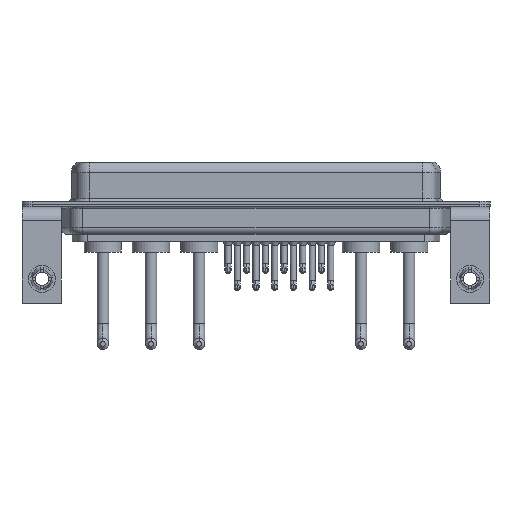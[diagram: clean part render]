
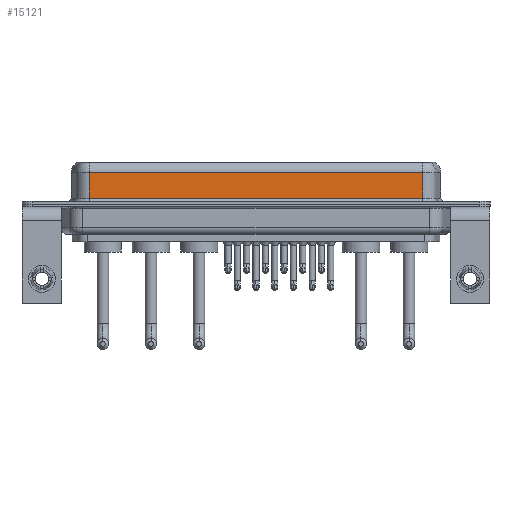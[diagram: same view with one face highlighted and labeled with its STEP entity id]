
A CAD part, front view. The second image highlights one B-rep face of the part: STEP entity #15121.
In plain terms, the highlighted planar face has unit normal (0, -1, 0).
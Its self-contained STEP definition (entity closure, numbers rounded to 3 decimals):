
#917 = FACE_OUTER_BOUND ( 'NONE', #13587, .T. ) ;
#1023 = VERTEX_POINT ( 'NONE', #16857 ) ;
#1134 = DIRECTION ( 'NONE',  ( 0., 1., 0. ) ) ;
#1253 = DIRECTION ( 'NONE',  ( 1., 0., 0. ) ) ;
#2992 = ORIENTED_EDGE ( 'NONE', *, *, #10327, .T. ) ;
#4061 = ORIENTED_EDGE ( 'NONE', *, *, #21674, .T. ) ;
#4792 = EDGE_CURVE ( 'NONE', #5984, #1023, #22410, .T. ) ;
#5480 = LINE ( 'NONE', #7325, #22406 ) ;
#5984 = VERTEX_POINT ( 'NONE', #9066 ) ;
#6277 = ORIENTED_EDGE ( 'NONE', *, *, #4792, .T. ) ;
#6581 = DIRECTION ( 'NONE',  ( -1., 0., 0. ) ) ;
#6910 = VECTOR ( 'NONE', #1253, 1000. ) ;
#7325 = CARTESIAN_POINT ( 'NONE',  ( 7.038, -3.95, 6.4 ) ) ;
#7396 = VERTEX_POINT ( 'NONE', #12749 ) ;
#7765 = PLANE ( 'NONE',  #15214 ) ;
#9066 = CARTESIAN_POINT ( 'NONE',  ( 7.038, -3.95, 0.9 ) ) ;
#10327 = EDGE_CURVE ( 'NONE', #20169, #7396, #18298, .T. ) ;
#10400 = VECTOR ( 'NONE', #19873, 1000. ) ;
#11409 = CARTESIAN_POINT ( 'NONE',  ( 56.462, -3.95, 4.65 ) ) ;
#11547 = CARTESIAN_POINT ( 'NONE',  ( 56.462, -3.95, 0.9 ) ) ;
#11805 = CARTESIAN_POINT ( 'NONE',  ( 56.462, -3.95, 4.65 ) ) ;
#12749 = CARTESIAN_POINT ( 'NONE',  ( 7.038, -3.95, 4.65 ) ) ;
#12929 = CARTESIAN_POINT ( 'NONE',  ( 56.462, -3.95, 6.4 ) ) ;
#13132 = ORIENTED_EDGE ( 'NONE', *, *, #15616, .F. ) ;
#13549 = VECTOR ( 'NONE', #6581, 1000. ) ;
#13587 = EDGE_LOOP ( 'NONE', ( #13132, #2992, #4061, #6277 ) ) ;
#14337 = DIRECTION ( 'NONE',  ( 0., 0., -1. ) ) ;
#14517 = CARTESIAN_POINT ( 'NONE',  ( 56.462, -3.95, 6.4 ) ) ;
#15121 = ADVANCED_FACE ( 'NONE', ( #917 ), #7765, .F. ) ;
#15214 = AXIS2_PLACEMENT_3D ( 'NONE', #12929, #1134, #18542 ) ;
#15616 = EDGE_CURVE ( 'NONE', #20169, #1023, #21579, .T. ) ;
#16857 = CARTESIAN_POINT ( 'NONE',  ( 56.462, -3.95, 0.9 ) ) ;
#18298 = LINE ( 'NONE', #11409, #13549 ) ;
#18542 = DIRECTION ( 'NONE',  ( 0., 0., 1. ) ) ;
#19873 = DIRECTION ( 'NONE',  ( 0., 0., -1. ) ) ;
#20169 = VERTEX_POINT ( 'NONE', #11805 ) ;
#21579 = LINE ( 'NONE', #14517, #10400 ) ;
#21674 = EDGE_CURVE ( 'NONE', #7396, #5984, #5480, .T. ) ;
#22406 = VECTOR ( 'NONE', #14337, 1000. ) ;
#22410 = LINE ( 'NONE', #11547, #6910 ) ;
